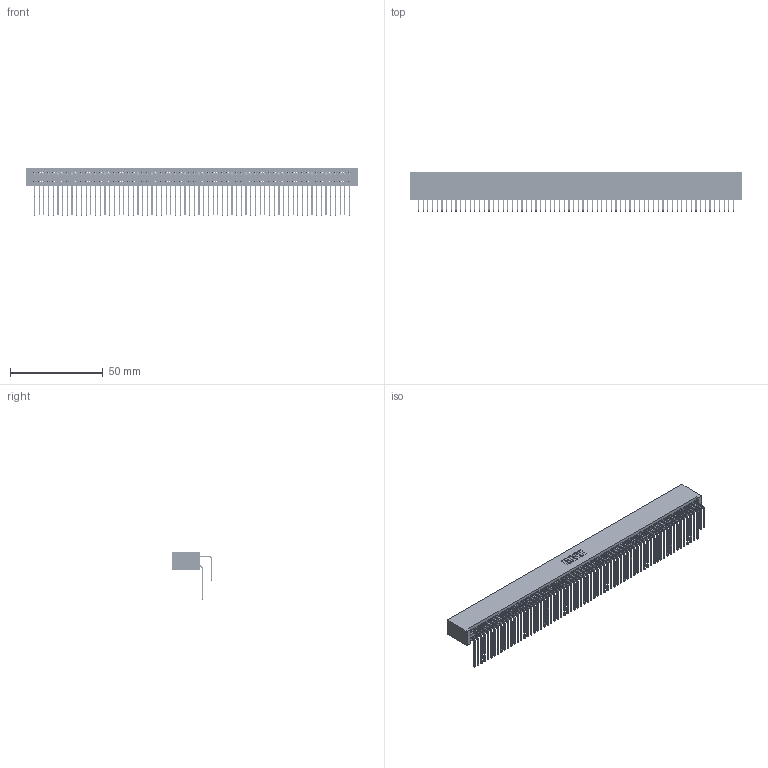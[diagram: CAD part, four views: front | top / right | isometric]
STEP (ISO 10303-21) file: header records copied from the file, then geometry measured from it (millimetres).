
FILE_DESCRIPTION (( 'STEP AP203' ), '1' );
FILE_NAME ('395-136-558-201.STEP', '2019-10-29T17:49:44', ( '' ), ( '' ), 'SwSTEP 2.0', 'SolidWorks 2016', '' );
FILE_SCHEMA (( 'CONFIG_CONTROL_DESIGN' ));
Length unit declared in the file: inch
Products named in the file (4): 345 Part_No Mounting Lugs; 345-292-001_558 559 Tail - 1; 345-292-001_558 Tail - 2; 395-136-558-201
Assembly tree (137 placements, depth 2):
  395-136-558-201
    345 Part_No Mounting Lugs
    345-292-001_558 559 Tail - 1  x68
    345-292-001_558 Tail - 2  x68
Bounding box: 179.32 x 21.83 x 25.53 mm (x, y, z)
Volume: 19061.5 mm3; surface area: 32672.2 mm2
Topology: 137 solids, 137 shells, 7190 faces, 21397 edges, 14082 vertices
Faces by surface type: plane 4836, cylinder 2354
Entity records: 51229 total; most frequent: CARTESIAN_POINT 8607, ORIENTED_EDGE 8490, DIRECTION 7525, EDGE_CURVE 4245, VECTOR 3809, LINE 3809, VERTEX_POINT 2826, AXIS2_PLACEMENT_3D 1858
